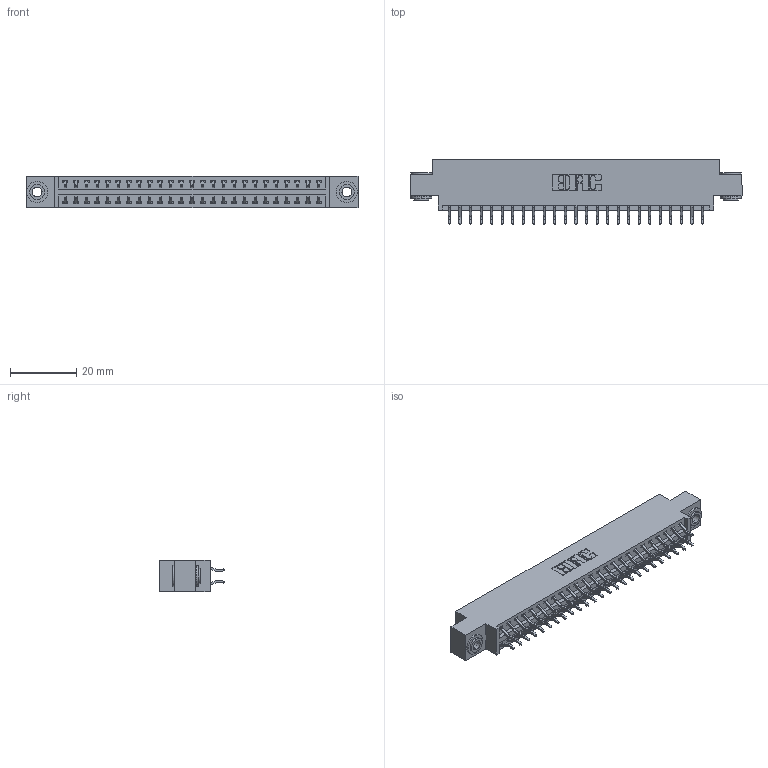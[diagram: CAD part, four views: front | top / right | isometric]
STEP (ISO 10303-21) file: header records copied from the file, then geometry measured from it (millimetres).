
FILE_DESCRIPTION (( 'STEP AP203' ), '1' );
FILE_NAME ('346-050-556-803.STEP', '2018-08-27T22:43:47', ( '' ), ( '' ), 'SwSTEP 2.0', 'SolidWorks 2016', '' );
FILE_SCHEMA (( 'CONFIG_CONTROL_DESIGN' ));
Length unit declared in the file: inch
Products named in the file (4): 345-292-001_556 Tail; 345-250-002_345-250-002-102; 346-050-556-803; 346 Part_0.170 Offset - 0.156 Dia-TH
Assembly tree (53 placements, depth 2):
  346-050-556-803
    346 Part_0.170 Offset - 0.156 Dia-TH
    345-292-001_556 Tail  x50
    345-250-002_345-250-002-102  x2
Bounding box: 99.95 x 19.57 x 9.4 mm (x, y, z)
Volume: 9477 mm3; surface area: 13107 mm2
Topology: 53 solids, 53 shells, 3064 faces, 9067 edges, 5974 vertices
Faces by surface type: plane 2040, cylinder 1016, cone 8
Entity records: 19606 total; most frequent: CARTESIAN_POINT 3247, ORIENTED_EDGE 3162, DIRECTION 2931, EDGE_CURVE 1581, LINE 1317, VECTOR 1317, VERTEX_POINT 1050, AXIS2_PLACEMENT_3D 807
